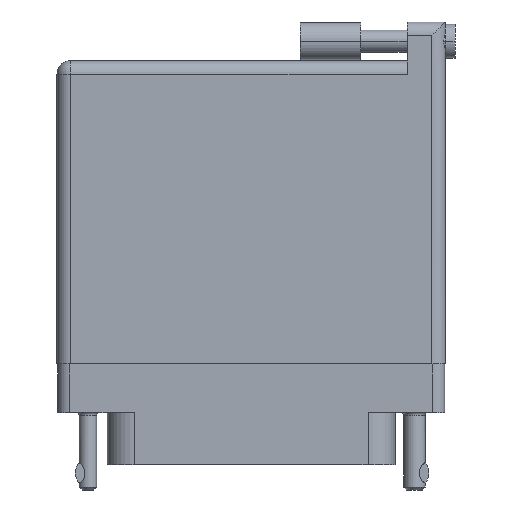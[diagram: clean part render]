
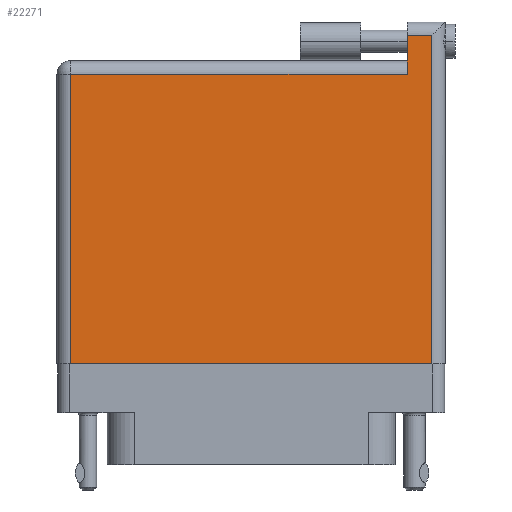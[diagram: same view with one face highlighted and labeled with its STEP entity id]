
A CAD part, front view. The second image highlights one B-rep face of the part: STEP entity #22271.
In plain terms, the highlighted face is planar.
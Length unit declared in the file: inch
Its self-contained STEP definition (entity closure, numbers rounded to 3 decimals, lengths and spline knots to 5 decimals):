
#304 = FACE_OUTER_BOUND ( 'NONE', #37187, .T. ) ;
#1014 = EDGE_CURVE ( 'NONE', #30819, #36847, #25588, .T. ) ;
#1334 = DIRECTION ( 'NONE',  ( -1., 0., 0. ) ) ;
#2101 = CARTESIAN_POINT ( 'NONE',  ( 0.807, 1.666, 0.4495 ) ) ;
#2671 = ORIENTED_EDGE ( 'NONE', *, *, #44542, .T. ) ;
#3366 = DIRECTION ( 'NONE',  ( -1., 0., 0. ) ) ;
#3440 = DIRECTION ( 'NONE',  ( -1., 0., 0. ) ) ;
#3512 = CARTESIAN_POINT ( 'NONE',  ( 0.807, 1.396, 0.4495 ) ) ;
#6249 = LINE ( 'NONE', #43527, #17532 ) ;
#6365 = ORIENTED_EDGE ( 'NONE', *, *, #14713, .T. ) ;
#6488 = CARTESIAN_POINT ( 'NONE',  ( 0.934, 1.596, 0.4495 ) ) ;
#8404 = CARTESIAN_POINT ( 'NONE',  ( -1.004, -0.1, 0.4495 ) ) ;
#8727 = DIRECTION ( 'NONE',  ( 1., 0., 0. ) ) ;
#8822 = CARTESIAN_POINT ( 'NONE',  ( 0.807, 1.596, 0.4495 ) ) ;
#10514 = DIRECTION ( 'NONE',  ( 0., 1., 0. ) ) ;
#14713 = EDGE_CURVE ( 'NONE', #36163, #34777, #45630, .T. ) ;
#16493 = DIRECTION ( 'NONE',  ( 0., -1., 0. ) ) ;
#17532 = VECTOR ( 'NONE', #16493, 39.37008 ) ;
#17790 = LINE ( 'NONE', #25559, #36770 ) ;
#18133 = CARTESIAN_POINT ( 'NONE',  ( 0.934, 1.666, 0.4495 ) ) ;
#18618 = LINE ( 'NONE', #29627, #42918 ) ;
#19254 = CARTESIAN_POINT ( 'NONE',  ( 0.934, -0.1, 0.4495 ) ) ;
#22271 = ADVANCED_FACE ( 'NONE', ( #304 ), #38773, .F. ) ;
#23040 = ORIENTED_EDGE ( 'NONE', *, *, #1014, .T. ) ;
#23236 = VECTOR ( 'NONE', #10514, 39.37008 ) ;
#25559 = CARTESIAN_POINT ( 'NONE',  ( -1.004, 1.596, 0.4495 ) ) ;
#25588 = LINE ( 'NONE', #2101, #29153 ) ;
#27623 = DIRECTION ( 'NONE',  ( 0., 0., -1. ) ) ;
#27717 = ORIENTED_EDGE ( 'NONE', *, *, #30451, .T. ) ;
#29153 = VECTOR ( 'NONE', #46983, 39.37008 ) ;
#29231 = EDGE_CURVE ( 'NONE', #34777, #40656, #33366, .T. ) ;
#29245 = CARTESIAN_POINT ( 'NONE',  ( -0.934, 1.396, 0.4495 ) ) ;
#29627 = CARTESIAN_POINT ( 'NONE',  ( -1.004, 1.396, 0.4495 ) ) ;
#30451 = EDGE_CURVE ( 'NONE', #40656, #30819, #17790, .T. ) ;
#30819 = VERTEX_POINT ( 'NONE', #8822 ) ;
#33366 = LINE ( 'NONE', #18133, #23236 ) ;
#34777 = VERTEX_POINT ( 'NONE', #19254 ) ;
#36163 = VERTEX_POINT ( 'NONE', #48132 ) ;
#36770 = VECTOR ( 'NONE', #3366, 39.37008 ) ;
#36847 = VERTEX_POINT ( 'NONE', #3512 ) ;
#37187 = EDGE_LOOP ( 'NONE', ( #6365, #41841, #27717, #23040, #41812, #2671 ) ) ;
#38640 = VERTEX_POINT ( 'NONE', #29245 ) ;
#38773 = PLANE ( 'NONE',  #38848 ) ;
#38848 = AXIS2_PLACEMENT_3D ( 'NONE', #39259, #27623, #1334 ) ;
#39259 = CARTESIAN_POINT ( 'NONE',  ( -1.004, 1.466, 0.4495 ) ) ;
#39743 = VECTOR ( 'NONE', #8727, 39.37008 ) ;
#40656 = VERTEX_POINT ( 'NONE', #6488 ) ;
#41812 = ORIENTED_EDGE ( 'NONE', *, *, #45655, .T. ) ;
#41841 = ORIENTED_EDGE ( 'NONE', *, *, #29231, .T. ) ;
#42918 = VECTOR ( 'NONE', #3440, 39.37008 ) ;
#43527 = CARTESIAN_POINT ( 'NONE',  ( -0.934, -0.1, 0.4495 ) ) ;
#44542 = EDGE_CURVE ( 'NONE', #38640, #36163, #6249, .T. ) ;
#45630 = LINE ( 'NONE', #8404, #39743 ) ;
#45655 = EDGE_CURVE ( 'NONE', #36847, #38640, #18618, .T. ) ;
#46983 = DIRECTION ( 'NONE',  ( 0., -1., 0. ) ) ;
#48132 = CARTESIAN_POINT ( 'NONE',  ( -0.934, -0.1, 0.4495 ) ) ;
